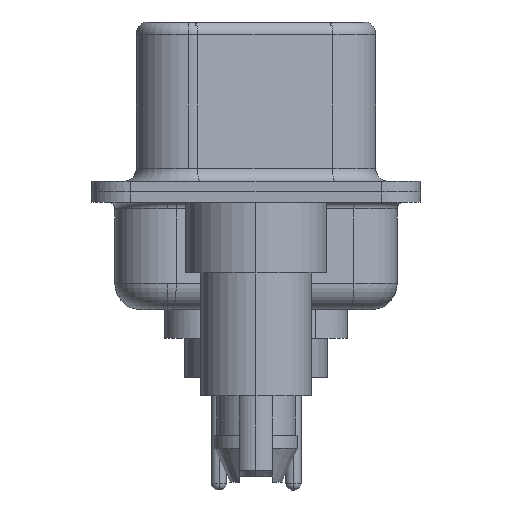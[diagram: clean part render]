
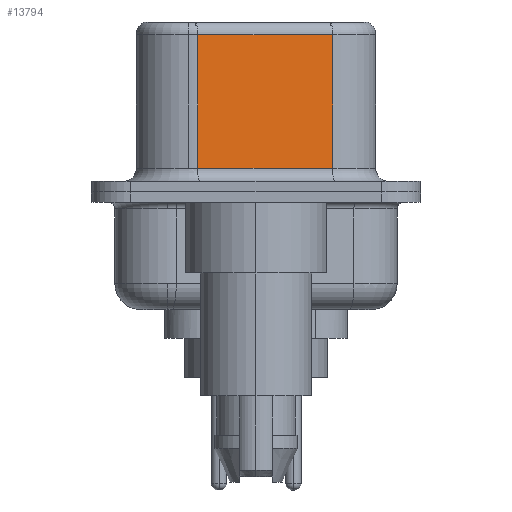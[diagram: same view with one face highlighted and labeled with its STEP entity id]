
A CAD part, left-side view. The second image highlights one B-rep face of the part: STEP entity #13794.
In plain terms, the highlighted planar face has unit normal (-0.985, -0.174, 0).
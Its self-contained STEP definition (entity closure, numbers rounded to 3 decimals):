
#1172 = VERTEX_POINT ( 'NONE', #10888 ) ;
#2273 = ORIENTED_EDGE ( 'NONE', *, *, #21145, .T. ) ;
#5257 = CARTESIAN_POINT ( 'NONE',  ( 4.58, -2.927, 6.02 ) ) ;
#5744 = CARTESIAN_POINT ( 'NONE',  ( 3.67, 2.233, 0.9 ) ) ;
#6538 = ORIENTED_EDGE ( 'NONE', *, *, #17036, .F. ) ;
#6861 = VECTOR ( 'NONE', #13347, 1000. ) ;
#6936 = DIRECTION ( 'NONE',  ( 0.174, -0.985, 0. ) ) ;
#6941 = VERTEX_POINT ( 'NONE', #5257 ) ;
#6992 = LINE ( 'NONE', #17555, #16635 ) ;
#7194 = ORIENTED_EDGE ( 'NONE', *, *, #18591, .T. ) ;
#7391 = EDGE_LOOP ( 'NONE', ( #6538, #7194, #2273, #25076 ) ) ;
#8178 = DIRECTION ( 'NONE',  ( 0.985, 0.174, 0. ) ) ;
#9636 = VECTOR ( 'NONE', #15230, 1000. ) ;
#10888 = CARTESIAN_POINT ( 'NONE',  ( 3.67, 2.233, 6.02 ) ) ;
#12370 = LINE ( 'NONE', #23434, #6861 ) ;
#13347 = DIRECTION ( 'NONE',  ( 0., 0., -1. ) ) ;
#13794 = ADVANCED_FACE ( 'NONE', ( #17939 ), #18402, .F. ) ;
#15230 = DIRECTION ( 'NONE',  ( 0., 0., -1. ) ) ;
#16635 = VECTOR ( 'NONE', #19593, 1000. ) ;
#17036 = EDGE_CURVE ( 'NONE', #6941, #23126, #25176, .T. ) ;
#17275 = CARTESIAN_POINT ( 'NONE',  ( 4.58, -2.927, 0.9 ) ) ;
#17555 = CARTESIAN_POINT ( 'NONE',  ( 4.58, -2.927, 6.02 ) ) ;
#17939 = FACE_OUTER_BOUND ( 'NONE', #7391, .T. ) ;
#18402 = PLANE ( 'NONE',  #21788 ) ;
#18591 = EDGE_CURVE ( 'NONE', #6941, #1172, #6992, .T. ) ;
#19061 = LINE ( 'NONE', #17275, #23769 ) ;
#19593 = DIRECTION ( 'NONE',  ( -0.174, 0.985, 0. ) ) ;
#21080 = EDGE_CURVE ( 'NONE', #26121, #23126, #19061, .T. ) ;
#21145 = EDGE_CURVE ( 'NONE', #1172, #26121, #12370, .T. ) ;
#21223 = CARTESIAN_POINT ( 'NONE',  ( 4.58, -2.927, 6.52 ) ) ;
#21788 = AXIS2_PLACEMENT_3D ( 'NONE', #26381, #8178, #22446 ) ;
#22446 = DIRECTION ( 'NONE',  ( -0.174, 0.985, 0. ) ) ;
#23126 = VERTEX_POINT ( 'NONE', #24312 ) ;
#23434 = CARTESIAN_POINT ( 'NONE',  ( 3.67, 2.233, 6.52 ) ) ;
#23769 = VECTOR ( 'NONE', #6936, 1000. ) ;
#24312 = CARTESIAN_POINT ( 'NONE',  ( 4.58, -2.927, 0.9 ) ) ;
#25076 = ORIENTED_EDGE ( 'NONE', *, *, #21080, .T. ) ;
#25176 = LINE ( 'NONE', #21223, #9636 ) ;
#26121 = VERTEX_POINT ( 'NONE', #5744 ) ;
#26381 = CARTESIAN_POINT ( 'NONE',  ( 4.58, -2.927, 6.52 ) ) ;
